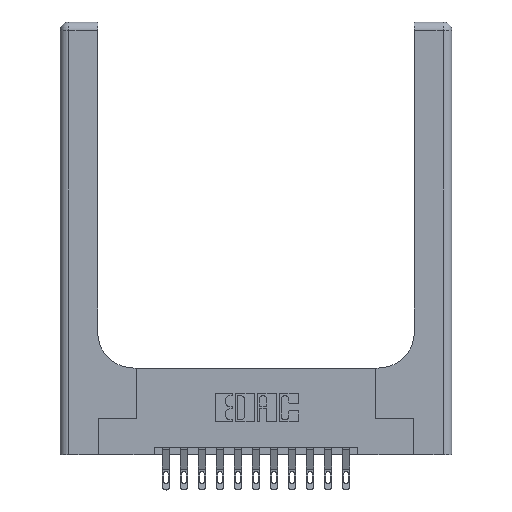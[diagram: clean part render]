
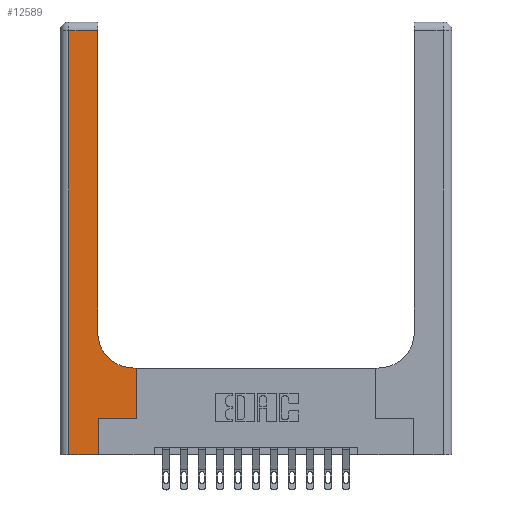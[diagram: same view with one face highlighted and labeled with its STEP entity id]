
A CAD part, top view. The second image highlights one B-rep face of the part: STEP entity #12589.
In plain terms, the highlighted planar face has unit normal (0, 0, 1).
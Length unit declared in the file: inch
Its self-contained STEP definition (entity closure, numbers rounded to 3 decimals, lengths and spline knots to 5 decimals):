
#215 = VERTEX_POINT ( 'NONE', #5740 ) ;
#742 = CARTESIAN_POINT ( 'NONE',  ( 0.265, 0.25, 0.37 ) ) ;
#941 = CARTESIAN_POINT ( 'NONE',  ( 0., 0., 0.37 ) ) ;
#1489 = LINE ( 'NONE', #6272, #8885 ) ;
#1614 = LINE ( 'NONE', #8901, #15705 ) ;
#1661 = VERTEX_POINT ( 'NONE', #3875 ) ;
#2206 = CARTESIAN_POINT ( 'NONE',  ( 0.528, 0.6, 0.37 ) ) ;
#2501 = DIRECTION ( 'NONE',  ( 0., 1., 0. ) ) ;
#2638 = FACE_OUTER_BOUND ( 'NONE', #12324, .T. ) ;
#2673 = ORIENTED_EDGE ( 'NONE', *, *, #16256, .T. ) ;
#2973 = ORIENTED_EDGE ( 'NONE', *, *, #6123, .T. ) ;
#3186 = VERTEX_POINT ( 'NONE', #4125 ) ;
#3660 = VERTEX_POINT ( 'NONE', #2206 ) ;
#3677 = CARTESIAN_POINT ( 'NONE',  ( 0.265, 0., 0.37 ) ) ;
#3875 = CARTESIAN_POINT ( 'NONE',  ( 0.26, 0.85, 0.37 ) ) ;
#4018 = LINE ( 'NONE', #4086, #12937 ) ;
#4086 = CARTESIAN_POINT ( 'NONE',  ( 0.06, 3., 0.37 ) ) ;
#4125 = CARTESIAN_POINT ( 'NONE',  ( 0.26, 2.94, 0.37 ) ) ;
#4155 = CARTESIAN_POINT ( 'NONE',  ( 0.51, 0.6, 0.37 ) ) ;
#4209 = ORIENTED_EDGE ( 'NONE', *, *, #4252, .T. ) ;
#4252 = EDGE_CURVE ( 'NONE', #215, #16295, #4346, .T. ) ;
#4286 = ORIENTED_EDGE ( 'NONE', *, *, #10882, .T. ) ;
#4346 = LINE ( 'NONE', #941, #4940 ) ;
#4559 = ORIENTED_EDGE ( 'NONE', *, *, #7777, .T. ) ;
#4726 = AXIS2_PLACEMENT_3D ( 'NONE', #9511, #5459, #13232 ) ;
#4806 = DIRECTION ( 'NONE',  ( 0., 1., 0. ) ) ;
#4940 = VECTOR ( 'NONE', #6332, 39.37008 ) ;
#5453 = EDGE_CURVE ( 'NONE', #16295, #14619, #8827, .T. ) ;
#5459 = DIRECTION ( 'NONE',  ( 0., 0., -1. ) ) ;
#5740 = CARTESIAN_POINT ( 'NONE',  ( 0.06, 0., 0.37 ) ) ;
#6123 = EDGE_CURVE ( 'NONE', #3660, #14588, #1614, .T. ) ;
#6272 = CARTESIAN_POINT ( 'NONE',  ( 0.26, 3., 0.37 ) ) ;
#6332 = DIRECTION ( 'NONE',  ( 1., 0., 0. ) ) ;
#6944 = VECTOR ( 'NONE', #15631, 39.37008 ) ;
#7197 = VECTOR ( 'NONE', #2501, 39.37008 ) ;
#7347 = VECTOR ( 'NONE', #4806, 39.37008 ) ;
#7479 = CIRCLE ( 'NONE', #13611, 0.25 ) ;
#7605 = LINE ( 'NONE', #7630, #7197 ) ;
#7630 = CARTESIAN_POINT ( 'NONE',  ( 0.528, 0.25, 0.37 ) ) ;
#7777 = EDGE_CURVE ( 'NONE', #14588, #1661, #7479, .T. ) ;
#8027 = DIRECTION ( 'NONE',  ( 0., -1., 0. ) ) ;
#8443 = EDGE_CURVE ( 'NONE', #11097, #215, #4018, .T. ) ;
#8812 = LINE ( 'NONE', #742, #13239 ) ;
#8827 = LINE ( 'NONE', #3677, #7347 ) ;
#8885 = VECTOR ( 'NONE', #10419, 39.37008 ) ;
#8901 = CARTESIAN_POINT ( 'NONE',  ( 0.26, 0.6, 0.37 ) ) ;
#9293 = CARTESIAN_POINT ( 'NONE',  ( 0.265, 0., 0.37 ) ) ;
#9511 = CARTESIAN_POINT ( 'NONE',  ( 0., 3., 0.37 ) ) ;
#10419 = DIRECTION ( 'NONE',  ( 0., 1., 0. ) ) ;
#10437 = LINE ( 'NONE', #14296, #6944 ) ;
#10447 = CARTESIAN_POINT ( 'NONE',  ( 0.06, 2.94, 0.37 ) ) ;
#10882 = EDGE_CURVE ( 'NONE', #14619, #11485, #8812, .T. ) ;
#11018 = ORIENTED_EDGE ( 'NONE', *, *, #11389, .T. ) ;
#11097 = VERTEX_POINT ( 'NONE', #10447 ) ;
#11389 = EDGE_CURVE ( 'NONE', #3186, #11097, #10437, .T. ) ;
#11485 = VERTEX_POINT ( 'NONE', #14415 ) ;
#11555 = DIRECTION ( 'NONE',  ( -1., 0., 0. ) ) ;
#11593 = DIRECTION ( 'NONE',  ( 1., 0., 0. ) ) ;
#12324 = EDGE_LOOP ( 'NONE', ( #16510, #11018, #16478, #4209, #14005, #4286, #2673, #2973, #4559 ) ) ;
#12589 = ADVANCED_FACE ( 'NONE', ( #2638 ), #14612, .F. ) ;
#12937 = VECTOR ( 'NONE', #8027, 39.37008 ) ;
#13028 = CARTESIAN_POINT ( 'NONE',  ( 0.51, 0.85, 0.37 ) ) ;
#13232 = DIRECTION ( 'NONE',  ( -1., 0., 0. ) ) ;
#13239 = VECTOR ( 'NONE', #15238, 39.37008 ) ;
#13611 = AXIS2_PLACEMENT_3D ( 'NONE', #13028, #14347, #11593 ) ;
#14005 = ORIENTED_EDGE ( 'NONE', *, *, #5453, .T. ) ;
#14296 = CARTESIAN_POINT ( 'NONE',  ( 0., 2.94, 0.37 ) ) ;
#14347 = DIRECTION ( 'NONE',  ( 0., 0., -1. ) ) ;
#14415 = CARTESIAN_POINT ( 'NONE',  ( 0.528, 0.25, 0.37 ) ) ;
#14588 = VERTEX_POINT ( 'NONE', #4155 ) ;
#14612 = PLANE ( 'NONE',  #4726 ) ;
#14619 = VERTEX_POINT ( 'NONE', #15842 ) ;
#15238 = DIRECTION ( 'NONE',  ( 1., 0., 0. ) ) ;
#15555 = EDGE_CURVE ( 'NONE', #1661, #3186, #1489, .T. ) ;
#15631 = DIRECTION ( 'NONE',  ( -1., 0., 0. ) ) ;
#15705 = VECTOR ( 'NONE', #11555, 39.37008 ) ;
#15842 = CARTESIAN_POINT ( 'NONE',  ( 0.265, 0.25, 0.37 ) ) ;
#16256 = EDGE_CURVE ( 'NONE', #11485, #3660, #7605, .T. ) ;
#16295 = VERTEX_POINT ( 'NONE', #9293 ) ;
#16478 = ORIENTED_EDGE ( 'NONE', *, *, #8443, .T. ) ;
#16510 = ORIENTED_EDGE ( 'NONE', *, *, #15555, .T. ) ;
